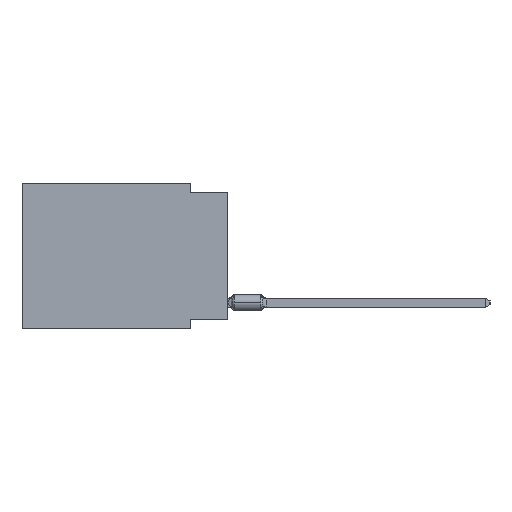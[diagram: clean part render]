
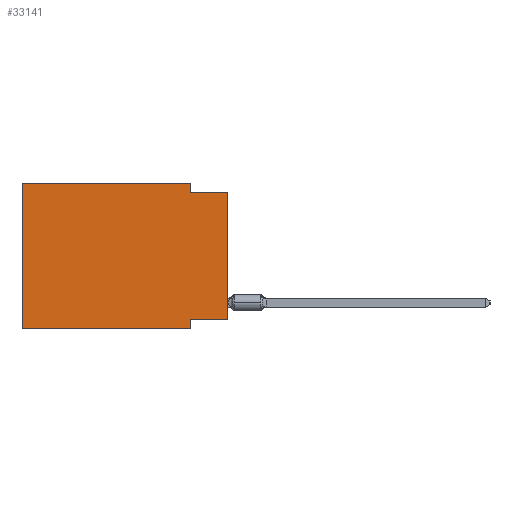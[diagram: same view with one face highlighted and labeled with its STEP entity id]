
A CAD part, left-side view. The second image highlights one B-rep face of the part: STEP entity #33141.
In plain terms, the highlighted planar face has unit normal (-1, 0, 0).
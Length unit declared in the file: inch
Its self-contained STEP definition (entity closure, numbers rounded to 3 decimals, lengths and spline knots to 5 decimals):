
#2426 = VERTEX_POINT ( 'NONE', #2581 ) ;
#2581 = CARTESIAN_POINT ( 'NONE',  ( 0., 0., -0.365 ) ) ;
#3121 = VERTEX_POINT ( 'NONE', #47982 ) ;
#3449 = ORIENTED_EDGE ( 'NONE', *, *, #53700, .F. ) ;
#4065 = CARTESIAN_POINT ( 'NONE',  ( 0., 0.55, 0. ) ) ;
#5354 = CARTESIAN_POINT ( 'NONE',  ( 0., 0., 0. ) ) ;
#6823 = ORIENTED_EDGE ( 'NONE', *, *, #62341, .F. ) ;
#8323 = VECTOR ( 'NONE', #34838, 39.37008 ) ;
#8386 = CARTESIAN_POINT ( 'NONE',  ( 0., 0.55, 0. ) ) ;
#8898 = EDGE_CURVE ( 'NONE', #31887, #63413, #55416, .T. ) ;
#9211 = VERTEX_POINT ( 'NONE', #19549 ) ;
#10943 = LINE ( 'NONE', #40457, #47140 ) ;
#12103 = EDGE_CURVE ( 'NONE', #9211, #63413, #39612, .T. ) ;
#12657 = AXIS2_PLACEMENT_3D ( 'NONE', #8386, #28351, #20946 ) ;
#15161 = VECTOR ( 'NONE', #38780, 39.37008 ) ;
#15531 = VECTOR ( 'NONE', #50474, 39.37008 ) ;
#15699 = ORIENTED_EDGE ( 'NONE', *, *, #8898, .F. ) ;
#17107 = CARTESIAN_POINT ( 'NONE',  ( 0., 0.1, -0.025 ) ) ;
#18311 = DIRECTION ( 'NONE',  ( 0., -1., 0. ) ) ;
#19549 = CARTESIAN_POINT ( 'NONE',  ( 0., 0.55, -0.39 ) ) ;
#20076 = DIRECTION ( 'NONE',  ( 0., 0., 1. ) ) ;
#20946 = DIRECTION ( 'NONE',  ( 0., 0., -1. ) ) ;
#22730 = CARTESIAN_POINT ( 'NONE',  ( 0., 0., -0.365 ) ) ;
#25129 = CARTESIAN_POINT ( 'NONE',  ( 0., 0.55, 0. ) ) ;
#25841 = CARTESIAN_POINT ( 'NONE',  ( 0., 0.1, -0.39 ) ) ;
#27174 = VECTOR ( 'NONE', #20076, 39.37008 ) ;
#28351 = DIRECTION ( 'NONE',  ( 1., 0., 0. ) ) ;
#28462 = CARTESIAN_POINT ( 'NONE',  ( 0., 0.55, -0.39 ) ) ;
#30050 = ORIENTED_EDGE ( 'NONE', *, *, #12103, .T. ) ;
#30586 = EDGE_LOOP ( 'NONE', ( #59441, #59653, #3449, #31457, #32851, #30050, #15699, #6823 ) ) ;
#31457 = ORIENTED_EDGE ( 'NONE', *, *, #59107, .F. ) ;
#31887 = VERTEX_POINT ( 'NONE', #37859 ) ;
#32115 = EDGE_CURVE ( 'NONE', #35148, #40187, #10943, .T. ) ;
#32851 = ORIENTED_EDGE ( 'NONE', *, *, #43904, .F. ) ;
#33141 = ADVANCED_FACE ( 'NONE', ( #58254 ), #53322, .F. ) ;
#34838 = DIRECTION ( 'NONE',  ( 0., 0., -1. ) ) ;
#35148 = VERTEX_POINT ( 'NONE', #17107 ) ;
#37859 = CARTESIAN_POINT ( 'NONE',  ( 0., 0.1, -0.365 ) ) ;
#38780 = DIRECTION ( 'NONE',  ( 0., 0., 1. ) ) ;
#39612 = LINE ( 'NONE', #28462, #46494 ) ;
#40187 = VERTEX_POINT ( 'NONE', #55032 ) ;
#40457 = CARTESIAN_POINT ( 'NONE',  ( 0., 0., -0.025 ) ) ;
#42758 = VERTEX_POINT ( 'NONE', #57086 ) ;
#43745 = LINE ( 'NONE', #22730, #64265 ) ;
#43904 = EDGE_CURVE ( 'NONE', #9211, #42758, #44385, .T. ) ;
#44385 = LINE ( 'NONE', #4065, #15161 ) ;
#45165 = DIRECTION ( 'NONE',  ( 0., -1., 0. ) ) ;
#46494 = VECTOR ( 'NONE', #18311, 39.37008 ) ;
#47140 = VECTOR ( 'NONE', #50003, 39.37008 ) ;
#47982 = CARTESIAN_POINT ( 'NONE',  ( 0., 0.1, 0. ) ) ;
#48354 = DIRECTION ( 'NONE',  ( 0., 1., 0. ) ) ;
#49629 = LINE ( 'NONE', #54568, #8323 ) ;
#49785 = EDGE_CURVE ( 'NONE', #2426, #40187, #64717, .T. ) ;
#50003 = DIRECTION ( 'NONE',  ( 0., -1., 0. ) ) ;
#50077 = LINE ( 'NONE', #25129, #59982 ) ;
#50474 = DIRECTION ( 'NONE',  ( 0., 0., -1. ) ) ;
#53322 = PLANE ( 'NONE',  #12657 ) ;
#53700 = EDGE_CURVE ( 'NONE', #3121, #35148, #49629, .T. ) ;
#54568 = CARTESIAN_POINT ( 'NONE',  ( 0., 0.1, 0. ) ) ;
#55032 = CARTESIAN_POINT ( 'NONE',  ( 0., 0., -0.025 ) ) ;
#55416 = LINE ( 'NONE', #60335, #15531 ) ;
#57086 = CARTESIAN_POINT ( 'NONE',  ( 0., 0.55, 0. ) ) ;
#58254 = FACE_OUTER_BOUND ( 'NONE', #30586, .T. ) ;
#59107 = EDGE_CURVE ( 'NONE', #42758, #3121, #50077, .T. ) ;
#59441 = ORIENTED_EDGE ( 'NONE', *, *, #49785, .T. ) ;
#59653 = ORIENTED_EDGE ( 'NONE', *, *, #32115, .F. ) ;
#59982 = VECTOR ( 'NONE', #45165, 39.37008 ) ;
#60335 = CARTESIAN_POINT ( 'NONE',  ( 0., 0.1, -0.39 ) ) ;
#62341 = EDGE_CURVE ( 'NONE', #2426, #31887, #43745, .T. ) ;
#63413 = VERTEX_POINT ( 'NONE', #25841 ) ;
#64265 = VECTOR ( 'NONE', #48354, 39.37008 ) ;
#64717 = LINE ( 'NONE', #5354, #27174 ) ;
